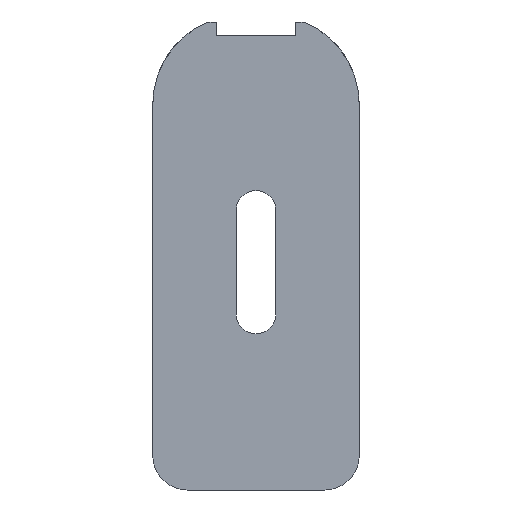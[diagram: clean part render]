
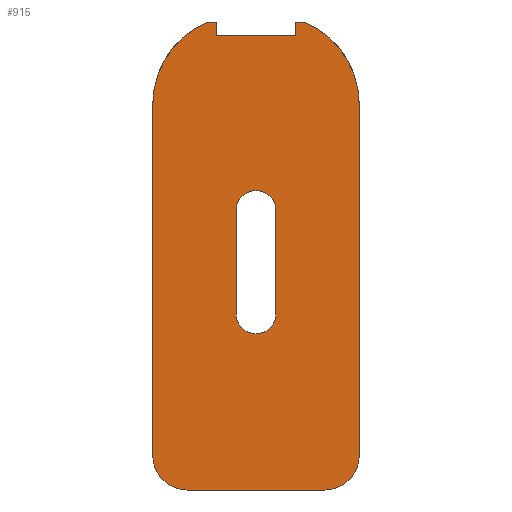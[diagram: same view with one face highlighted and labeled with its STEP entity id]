
A CAD part, front view. The second image highlights one B-rep face of the part: STEP entity #915.
In plain terms, the highlighted planar face has unit normal (0, -1, 0).
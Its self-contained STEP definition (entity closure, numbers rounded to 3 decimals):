
#24 = LINE ( 'NONE', #573, #168 ) ;
#28 = DIRECTION ( 'NONE',  ( 1., 0., 0. ) ) ;
#32 = CARTESIAN_POINT ( 'NONE',  ( -2.9, 0., 6.6 ) ) ;
#39 = ORIENTED_EDGE ( 'NONE', *, *, #748, .T. ) ;
#74 = DIRECTION ( 'NONE',  ( 0., -1., 0. ) ) ;
#86 = CARTESIAN_POINT ( 'NONE',  ( 15., 0., 22. ) ) ;
#94 = ORIENTED_EDGE ( 'NONE', *, *, #1219, .F. ) ;
#96 = LINE ( 'NONE', #1454, #264 ) ;
#102 = VERTEX_POINT ( 'NONE', #391 ) ;
#103 = CARTESIAN_POINT ( 'NONE',  ( 0., 0., 6.6 ) ) ;
#110 = VERTEX_POINT ( 'NONE', #1403 ) ;
#113 = DIRECTION ( 'NONE',  ( 0., 0., 1. ) ) ;
#127 = EDGE_CURVE ( 'NONE', #558, #360, #1394, .T. ) ;
#130 = LINE ( 'NONE', #262, #936 ) ;
#166 = CARTESIAN_POINT ( 'NONE',  ( 0., 0., -8.4 ) ) ;
#168 = VECTOR ( 'NONE', #1157, 1000. ) ;
#171 = VECTOR ( 'NONE', #1199, 1000. ) ;
#186 = VERTEX_POINT ( 'NONE', #863 ) ;
#198 = VERTEX_POINT ( 'NONE', #767 ) ;
#213 = CIRCLE ( 'NONE', #1153, 13. ) ;
#216 = VERTEX_POINT ( 'NONE', #277 ) ;
#229 = EDGE_CURVE ( 'NONE', #1423, #984, #1130, .T. ) ;
#232 = CARTESIAN_POINT ( 'NONE',  ( -10., 0., -29. ) ) ;
#239 = CIRCLE ( 'NONE', #430, 13. ) ;
#249 = EDGE_CURVE ( 'NONE', #305, #894, #239, .T. ) ;
#262 = CARTESIAN_POINT ( 'NONE',  ( -5.75, 0., 32. ) ) ;
#264 = VECTOR ( 'NONE', #113, 1000. ) ;
#269 = DIRECTION ( 'NONE',  ( 0., 1., 0. ) ) ;
#270 = AXIS2_PLACEMENT_3D ( 'NONE', #166, #1399, #400 ) ;
#276 = CARTESIAN_POINT ( 'NONE',  ( -2.9, 0., -8.4 ) ) ;
#277 = CARTESIAN_POINT ( 'NONE',  ( 0., 0., 9.5 ) ) ;
#296 = CARTESIAN_POINT ( 'NONE',  ( -5.75, 0., 34. ) ) ;
#299 = ORIENTED_EDGE ( 'NONE', *, *, #864, .T. ) ;
#305 = VERTEX_POINT ( 'NONE', #86 ) ;
#306 = CARTESIAN_POINT ( 'NONE',  ( -5.75, 0., 34. ) ) ;
#310 = VECTOR ( 'NONE', #1217, 1000. ) ;
#324 = VERTEX_POINT ( 'NONE', #865 ) ;
#339 = CARTESIAN_POINT ( 'NONE',  ( -15., 0., 34. ) ) ;
#347 = EDGE_CURVE ( 'NONE', #216, #102, #1226, .T. ) ;
#348 = ORIENTED_EDGE ( 'NONE', *, *, #656, .T. ) ;
#352 = AXIS2_PLACEMENT_3D ( 'NONE', #1141, #1012, #1234 ) ;
#360 = VERTEX_POINT ( 'NONE', #1286 ) ;
#382 = VECTOR ( 'NONE', #744, 1000. ) ;
#389 = LINE ( 'NONE', #306, #641 ) ;
#390 = DIRECTION ( 'NONE',  ( 0., 0., -1. ) ) ;
#391 = CARTESIAN_POINT ( 'NONE',  ( 2.9, 0., 6.6 ) ) ;
#396 = DIRECTION ( 'NONE',  ( 0., 0., 1. ) ) ;
#400 = DIRECTION ( 'NONE',  ( 0., 0., 1. ) ) ;
#421 = EDGE_CURVE ( 'NONE', #1081, #562, #678, .T. ) ;
#429 = CIRCLE ( 'NONE', #757, 5. ) ;
#430 = AXIS2_PLACEMENT_3D ( 'NONE', #515, #837, #925 ) ;
#443 = ORIENTED_EDGE ( 'NONE', *, *, #461, .T. ) ;
#461 = EDGE_CURVE ( 'NONE', #562, #913, #130, .T. ) ;
#515 = CARTESIAN_POINT ( 'NONE',  ( 2., 0., 22. ) ) ;
#541 = VECTOR ( 'NONE', #28, 1000. ) ;
#554 = DIRECTION ( 'NONE',  ( 0., 1., 0. ) ) ;
#558 = VERTEX_POINT ( 'NONE', #611 ) ;
#562 = VERTEX_POINT ( 'NONE', #1051 ) ;
#568 = EDGE_CURVE ( 'NONE', #324, #198, #213, .T. ) ;
#573 = CARTESIAN_POINT ( 'NONE',  ( -15., 0., 34. ) ) ;
#576 = FACE_OUTER_BOUND ( 'NONE', #1431, .T. ) ;
#583 = VERTEX_POINT ( 'NONE', #296 ) ;
#590 = DIRECTION ( 'NONE',  ( 0., 0., -1. ) ) ;
#597 = AXIS2_PLACEMENT_3D ( 'NONE', #652, #269, #1163 ) ;
#606 = ORIENTED_EDGE ( 'NONE', *, *, #127, .T. ) ;
#611 = CARTESIAN_POINT ( 'NONE',  ( 10., 0., -34. ) ) ;
#615 = ORIENTED_EDGE ( 'NONE', *, *, #421, .T. ) ;
#627 = EDGE_CURVE ( 'NONE', #305, #360, #1296, .T. ) ;
#638 = DIRECTION ( 'NONE',  ( -1., 0., 0. ) ) ;
#641 = VECTOR ( 'NONE', #396, 1000. ) ;
#652 = CARTESIAN_POINT ( 'NONE',  ( 0., 0., 6.6 ) ) ;
#656 = EDGE_CURVE ( 'NONE', #913, #583, #389, .T. ) ;
#678 = LINE ( 'NONE', #872, #1183 ) ;
#684 = LINE ( 'NONE', #339, #310 ) ;
#710 = DIRECTION ( 'NONE',  ( -1., 0., 0. ) ) ;
#720 = EDGE_CURVE ( 'NONE', #984, #1161, #96, .T. ) ;
#733 = CARTESIAN_POINT ( 'NONE',  ( 15., 0., 34. ) ) ;
#744 = DIRECTION ( 'NONE',  ( 0., 0., -1. ) ) ;
#748 = EDGE_CURVE ( 'NONE', #102, #1423, #888, .T. ) ;
#751 = ORIENTED_EDGE ( 'NONE', *, *, #1311, .F. ) ;
#757 = AXIS2_PLACEMENT_3D ( 'NONE', #232, #896, #590 ) ;
#767 = CARTESIAN_POINT ( 'NONE',  ( -15., 0., 22. ) ) ;
#782 = EDGE_CURVE ( 'NONE', #1161, #216, #1107, .T. ) ;
#783 = ORIENTED_EDGE ( 'NONE', *, *, #720, .T. ) ;
#803 = ORIENTED_EDGE ( 'NONE', *, *, #627, .F. ) ;
#808 = LINE ( 'NONE', #1026, #541 ) ;
#821 = CARTESIAN_POINT ( 'NONE',  ( 2.9, 0., -8.4 ) ) ;
#837 = DIRECTION ( 'NONE',  ( 0., -1., 0. ) ) ;
#847 = ORIENTED_EDGE ( 'NONE', *, *, #1395, .F. ) ;
#863 = CARTESIAN_POINT ( 'NONE',  ( -15., 0., -29. ) ) ;
#864 = EDGE_CURVE ( 'NONE', #186, #110, #429, .T. ) ;
#865 = CARTESIAN_POINT ( 'NONE',  ( -7., 0., 34. ) ) ;
#870 = DIRECTION ( 'NONE',  ( 0., 0., 1. ) ) ;
#872 = CARTESIAN_POINT ( 'NONE',  ( 5.75, 0., 34. ) ) ;
#881 = CARTESIAN_POINT ( 'NONE',  ( 2.9, 0., -8.4 ) ) ;
#887 = ORIENTED_EDGE ( 'NONE', *, *, #782, .T. ) ;
#888 = LINE ( 'NONE', #881, #171 ) ;
#894 = VERTEX_POINT ( 'NONE', #1239 ) ;
#896 = DIRECTION ( 'NONE',  ( 0., -1., 0. ) ) ;
#913 = VERTEX_POINT ( 'NONE', #1018 ) ;
#915 = ADVANCED_FACE ( 'NONE', ( #576, #1363 ), #1257, .T. ) ;
#919 = ORIENTED_EDGE ( 'NONE', *, *, #568, .T. ) ;
#925 = DIRECTION ( 'NONE',  ( 0., 0., 1. ) ) ;
#926 = CARTESIAN_POINT ( 'NONE',  ( 5.75, 0., 34. ) ) ;
#936 = VECTOR ( 'NONE', #710, 1000. ) ;
#937 = CARTESIAN_POINT ( 'NONE',  ( -2., 0., 22. ) ) ;
#959 = ORIENTED_EDGE ( 'NONE', *, *, #1436, .F. ) ;
#973 = ORIENTED_EDGE ( 'NONE', *, *, #229, .T. ) ;
#984 = VERTEX_POINT ( 'NONE', #276 ) ;
#1012 = DIRECTION ( 'NONE',  ( 0., -1., 0. ) ) ;
#1018 = CARTESIAN_POINT ( 'NONE',  ( -5.75, 0., 32. ) ) ;
#1026 = CARTESIAN_POINT ( 'NONE',  ( -15., 0., 34. ) ) ;
#1051 = CARTESIAN_POINT ( 'NONE',  ( 5.75, 0., 32. ) ) ;
#1064 = AXIS2_PLACEMENT_3D ( 'NONE', #1085, #74, #1422 ) ;
#1079 = CARTESIAN_POINT ( 'NONE',  ( -15., 0., -34. ) ) ;
#1081 = VERTEX_POINT ( 'NONE', #926 ) ;
#1085 = CARTESIAN_POINT ( 'NONE',  ( 10., 0., -29. ) ) ;
#1095 = ORIENTED_EDGE ( 'NONE', *, *, #347, .T. ) ;
#1098 = LINE ( 'NONE', #1079, #1298 ) ;
#1107 = CIRCLE ( 'NONE', #1222, 2.9 ) ;
#1130 = CIRCLE ( 'NONE', #270, 2.9 ) ;
#1140 = EDGE_LOOP ( 'NONE', ( #973, #783, #887, #1095, #39 ) ) ;
#1141 = CARTESIAN_POINT ( 'NONE',  ( 0., 0., 0. ) ) ;
#1153 = AXIS2_PLACEMENT_3D ( 'NONE', #937, #1396, #390 ) ;
#1157 = DIRECTION ( 'NONE',  ( 0., 0., 1. ) ) ;
#1161 = VERTEX_POINT ( 'NONE', #32 ) ;
#1163 = DIRECTION ( 'NONE',  ( 0., 0., 1. ) ) ;
#1183 = VECTOR ( 'NONE', #1221, 1000. ) ;
#1199 = DIRECTION ( 'NONE',  ( 0., 0., -1. ) ) ;
#1217 = DIRECTION ( 'NONE',  ( 1., 0., 0. ) ) ;
#1219 = EDGE_CURVE ( 'NONE', #324, #583, #808, .T. ) ;
#1221 = DIRECTION ( 'NONE',  ( 0., 0., -1. ) ) ;
#1222 = AXIS2_PLACEMENT_3D ( 'NONE', #103, #554, #870 ) ;
#1226 = CIRCLE ( 'NONE', #597, 2.9 ) ;
#1234 = DIRECTION ( 'NONE',  ( 0., 0., -1. ) ) ;
#1239 = CARTESIAN_POINT ( 'NONE',  ( 7., 0., 34. ) ) ;
#1255 = ORIENTED_EDGE ( 'NONE', *, *, #249, .T. ) ;
#1257 = PLANE ( 'NONE',  #352 ) ;
#1286 = CARTESIAN_POINT ( 'NONE',  ( 15., 0., -29. ) ) ;
#1296 = LINE ( 'NONE', #733, #382 ) ;
#1298 = VECTOR ( 'NONE', #638, 1000. ) ;
#1311 = EDGE_CURVE ( 'NONE', #186, #198, #24, .T. ) ;
#1363 = FACE_BOUND ( 'NONE', #1140, .T. ) ;
#1394 = CIRCLE ( 'NONE', #1064, 5. ) ;
#1395 = EDGE_CURVE ( 'NONE', #1081, #894, #684, .T. ) ;
#1396 = DIRECTION ( 'NONE',  ( 0., -1., 0. ) ) ;
#1399 = DIRECTION ( 'NONE',  ( 0., 1., 0. ) ) ;
#1403 = CARTESIAN_POINT ( 'NONE',  ( -10., 0., -34. ) ) ;
#1422 = DIRECTION ( 'NONE',  ( 0., 0., -1. ) ) ;
#1423 = VERTEX_POINT ( 'NONE', #821 ) ;
#1431 = EDGE_LOOP ( 'NONE', ( #751, #299, #959, #606, #803, #1255, #847, #615, #443, #348, #94, #919 ) ) ;
#1436 = EDGE_CURVE ( 'NONE', #558, #110, #1098, .T. ) ;
#1454 = CARTESIAN_POINT ( 'NONE',  ( -2.9, 0., -8.4 ) ) ;
